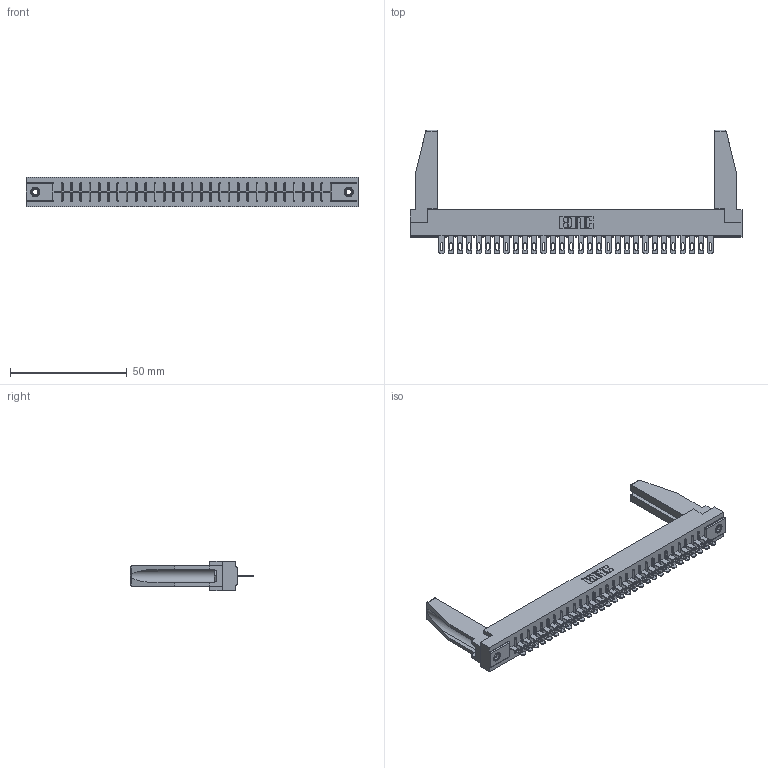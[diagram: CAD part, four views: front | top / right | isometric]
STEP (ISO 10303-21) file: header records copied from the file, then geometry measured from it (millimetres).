
FILE_DESCRIPTION (( 'STEP AP203' ), '1' );
FILE_NAME ('356-030-400-178.STEP', '2020-09-23T20:24:49', ( '' ), ( '' ), 'SwSTEP 2.0', 'SolidWorks 2020', '' );
FILE_SCHEMA (( 'CONFIG_CONTROL_DESIGN' ));
Length unit declared in the file: inch
Products named in the file (5): 306 Part_.156 Dia; 356-030-400-178; 307-220-078; 306-290-001_100; 345-250-001_345-250-001-102
Assembly tree (35 placements, depth 2):
  356-030-400-178
    306 Part_.156 Dia
    306-290-001_100  x30
    345-250-001_345-250-001-102  x2
    307-220-078  x2
Bounding box: 141.88 x 52.91 x 12.7 mm (x, y, z)
Volume: 19668.3 mm3; surface area: 20322.3 mm2
Topology: 35 solids, 35 shells, 2526 faces, 7096 edges, 4560 vertices
Faces by surface type: plane 1652, cylinder 738, sphere 120, cone 12, torus 4
Entity records: 32134 total; most frequent: CARTESIAN_POINT 5395, ORIENTED_EDGE 5306, DIRECTION 5273, EDGE_CURVE 2653, LINE 2069, VECTOR 2069, VERTEX_POINT 1682, AXIS2_PLACEMENT_3D 1602
